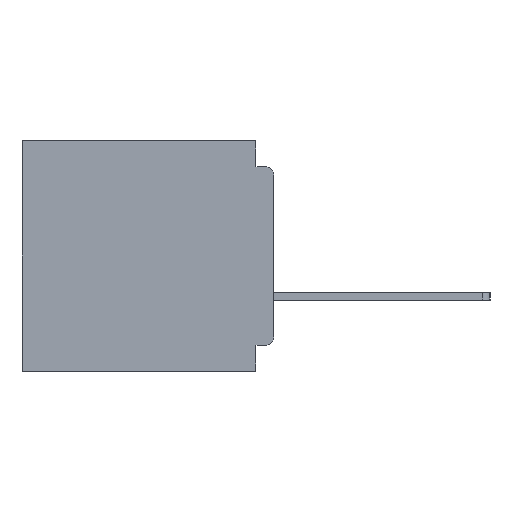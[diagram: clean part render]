
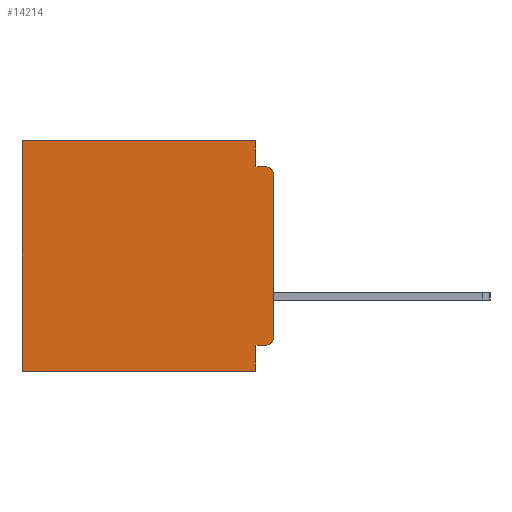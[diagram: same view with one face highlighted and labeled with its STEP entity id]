
A CAD part, left-side view. The second image highlights one B-rep face of the part: STEP entity #14214.
In plain terms, the highlighted planar face has unit normal (-1, 0, 0).
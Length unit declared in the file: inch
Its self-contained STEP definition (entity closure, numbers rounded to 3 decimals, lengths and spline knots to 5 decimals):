
#25 = AXIS2_PLACEMENT_3D ( 'NONE', #41969, #18144, #45909 ) ;
#77 = CARTESIAN_POINT ( 'NONE',  ( 0.3, 0.015, -0.355 ) ) ;
#136 = DIRECTION ( 'NONE',  ( 0., 1., 0. ) ) ;
#858 = EDGE_CURVE ( 'NONE', #23723, #43542, #17284, .T. ) ;
#912 = LINE ( 'NONE', #13211, #32664 ) ;
#1579 = EDGE_LOOP ( 'NONE', ( #31080, #39752, #45282, #42219, #45918, #2417, #49481, #12374, #32356, #23572 ) ) ;
#2417 = ORIENTED_EDGE ( 'NONE', *, *, #39962, .T. ) ;
#2495 = CARTESIAN_POINT ( 'NONE',  ( 0.3, 0.031, -0.355 ) ) ;
#3116 = CARTESIAN_POINT ( 'NONE',  ( 0.3, 0.031, -0.045 ) ) ;
#3132 = CARTESIAN_POINT ( 'NONE',  ( 0.3, 0.437, -0.4 ) ) ;
#3404 = LINE ( 'NONE', #33819, #44390 ) ;
#3557 = VECTOR ( 'NONE', #136, 39.37008 ) ;
#3785 = CARTESIAN_POINT ( 'NONE',  ( 0.3, 0., -0.34 ) ) ;
#4287 = DIRECTION ( 'NONE',  ( 0., 0., -1. ) ) ;
#5291 = CARTESIAN_POINT ( 'NONE',  ( 0.3, 0.031, 0. ) ) ;
#6004 = DIRECTION ( 'NONE',  ( 0., 1., 0. ) ) ;
#7715 = CARTESIAN_POINT ( 'NONE',  ( 0.3, 0., -0.06 ) ) ;
#9025 = EDGE_CURVE ( 'NONE', #11476, #26243, #3404, .T. ) ;
#10563 = DIRECTION ( 'NONE',  ( -1., 0., 0. ) ) ;
#11476 = VERTEX_POINT ( 'NONE', #77 ) ;
#11810 = DIRECTION ( 'NONE',  ( 0., 0., -1. ) ) ;
#12374 = ORIENTED_EDGE ( 'NONE', *, *, #34691, .F. ) ;
#13211 = CARTESIAN_POINT ( 'NONE',  ( 0.3, 0.031, -0.4 ) ) ;
#14214 = ADVANCED_FACE ( 'NONE', ( #47861 ), #20008, .F. ) ;
#14382 = EDGE_CURVE ( 'NONE', #11476, #43542, #49651, .T. ) ;
#17006 = AXIS2_PLACEMENT_3D ( 'NONE', #24016, #28063, #4287 ) ;
#17284 = LINE ( 'NONE', #42063, #37210 ) ;
#17502 = EDGE_CURVE ( 'NONE', #48475, #33200, #18464, .T. ) ;
#17971 = VECTOR ( 'NONE', #45896, 39.37008 ) ;
#18144 = DIRECTION ( 'NONE',  ( -1., 0., 0. ) ) ;
#18464 = LINE ( 'NONE', #5291, #29094 ) ;
#19730 = EDGE_CURVE ( 'NONE', #33200, #29745, #51222, .T. ) ;
#20008 = PLANE ( 'NONE',  #17006 ) ;
#21175 = VERTEX_POINT ( 'NONE', #47717 ) ;
#23572 = ORIENTED_EDGE ( 'NONE', *, *, #14382, .T. ) ;
#23723 = VERTEX_POINT ( 'NONE', #7715 ) ;
#24016 = CARTESIAN_POINT ( 'NONE',  ( 0.3, 0., -0.4 ) ) ;
#24873 = VERTEX_POINT ( 'NONE', #31761 ) ;
#25326 = LINE ( 'NONE', #37815, #33525 ) ;
#26086 = DIRECTION ( 'NONE',  ( 0., -1., 0. ) ) ;
#26243 = VERTEX_POINT ( 'NONE', #2495 ) ;
#26726 = CARTESIAN_POINT ( 'NONE',  ( 0.3, 0.031, 0. ) ) ;
#27455 = EDGE_CURVE ( 'NONE', #24873, #35659, #25326, .T. ) ;
#28063 = DIRECTION ( 'NONE',  ( 1., 0., 0. ) ) ;
#28996 = CARTESIAN_POINT ( 'NONE',  ( 0.3, 0.015, -0.045 ) ) ;
#29094 = VECTOR ( 'NONE', #44860, 39.37008 ) ;
#29745 = VERTEX_POINT ( 'NONE', #28996 ) ;
#30021 = DIRECTION ( 'NONE',  ( 0., 1., 0. ) ) ;
#30381 = VECTOR ( 'NONE', #26086, 39.37008 ) ;
#31080 = ORIENTED_EDGE ( 'NONE', *, *, #858, .F. ) ;
#31761 = CARTESIAN_POINT ( 'NONE',  ( 0.3, 0.031, -0.4 ) ) ;
#32356 = ORIENTED_EDGE ( 'NONE', *, *, #9025, .F. ) ;
#32664 = VECTOR ( 'NONE', #48846, 39.37008 ) ;
#33200 = VERTEX_POINT ( 'NONE', #3116 ) ;
#33342 = EDGE_CURVE ( 'NONE', #48475, #21175, #36557, .T. ) ;
#33525 = VECTOR ( 'NONE', #30021, 39.37008 ) ;
#33819 = CARTESIAN_POINT ( 'NONE',  ( 0.3, 0., -0.355 ) ) ;
#34391 = CARTESIAN_POINT ( 'NONE',  ( 0.3, 0.015, -0.06 ) ) ;
#34691 = EDGE_CURVE ( 'NONE', #26243, #24873, #912, .T. ) ;
#35659 = VERTEX_POINT ( 'NONE', #3132 ) ;
#36557 = LINE ( 'NONE', #47628, #3557 ) ;
#37210 = VECTOR ( 'NONE', #11810, 39.37008 ) ;
#37815 = CARTESIAN_POINT ( 'NONE',  ( 0.3, 0., -0.4 ) ) ;
#38145 = CARTESIAN_POINT ( 'NONE',  ( 0.3, 0.437, -0.4 ) ) ;
#38366 = DIRECTION ( 'NONE',  ( 0., 0., -1. ) ) ;
#39752 = ORIENTED_EDGE ( 'NONE', *, *, #43873, .T. ) ;
#39962 = EDGE_CURVE ( 'NONE', #21175, #35659, #50724, .T. ) ;
#41969 = CARTESIAN_POINT ( 'NONE',  ( 0.3, 0.015, -0.34 ) ) ;
#42063 = CARTESIAN_POINT ( 'NONE',  ( 0.3, 0., -0.4 ) ) ;
#42219 = ORIENTED_EDGE ( 'NONE', *, *, #17502, .F. ) ;
#43542 = VERTEX_POINT ( 'NONE', #3785 ) ;
#43873 = EDGE_CURVE ( 'NONE', #23723, #29745, #49629, .T. ) ;
#44390 = VECTOR ( 'NONE', #6004, 39.37008 ) ;
#44860 = DIRECTION ( 'NONE',  ( 0., 0., -1. ) ) ;
#45282 = ORIENTED_EDGE ( 'NONE', *, *, #19730, .F. ) ;
#45892 = CARTESIAN_POINT ( 'NONE',  ( 0.3, 0., -0.045 ) ) ;
#45896 = DIRECTION ( 'NONE',  ( 0., 0., -1. ) ) ;
#45909 = DIRECTION ( 'NONE',  ( 0., 0., -1. ) ) ;
#45918 = ORIENTED_EDGE ( 'NONE', *, *, #33342, .T. ) ;
#47628 = CARTESIAN_POINT ( 'NONE',  ( 0.3, 0., 0. ) ) ;
#47717 = CARTESIAN_POINT ( 'NONE',  ( 0.3, 0.437, 0. ) ) ;
#47861 = FACE_OUTER_BOUND ( 'NONE', #1579, .T. ) ;
#48475 = VERTEX_POINT ( 'NONE', #26726 ) ;
#48846 = DIRECTION ( 'NONE',  ( 0., 0., -1. ) ) ;
#49481 = ORIENTED_EDGE ( 'NONE', *, *, #27455, .F. ) ;
#49571 = AXIS2_PLACEMENT_3D ( 'NONE', #34391, #10563, #38366 ) ;
#49629 = CIRCLE ( 'NONE', #49571, 0.015 ) ;
#49651 = CIRCLE ( 'NONE', #25, 0.015 ) ;
#50724 = LINE ( 'NONE', #38145, #17971 ) ;
#51222 = LINE ( 'NONE', #45892, #30381 ) ;
